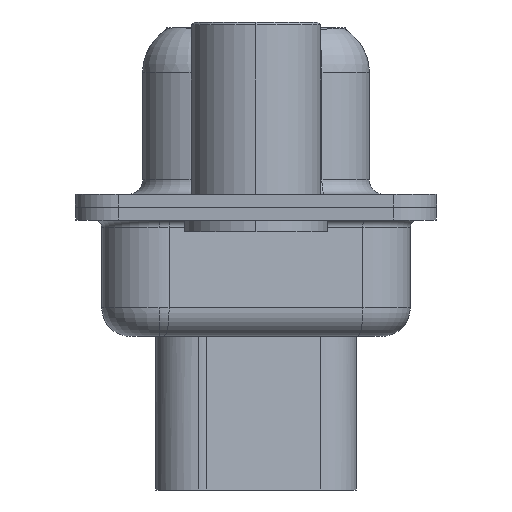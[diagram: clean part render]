
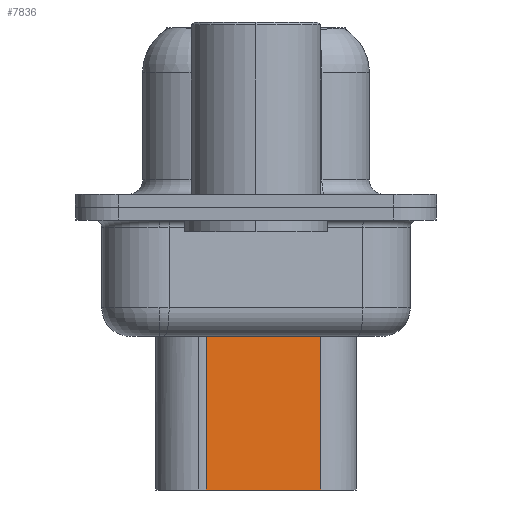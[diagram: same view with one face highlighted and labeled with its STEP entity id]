
A CAD part, left-side view. The second image highlights one B-rep face of the part: STEP entity #7836.
In plain terms, the highlighted planar face has unit normal (-0.985, -0.174, 0).
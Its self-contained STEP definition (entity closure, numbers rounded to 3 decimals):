
#334 = VECTOR ( 'NONE', #9859, 1000. ) ;
#618 = DIRECTION ( 'NONE',  ( 0.174, -0.985, 0. ) ) ;
#912 = VERTEX_POINT ( 'NONE', #12681 ) ;
#1191 = CARTESIAN_POINT ( 'NONE',  ( 5.224, -2.26, -9.85 ) ) ;
#1565 = EDGE_CURVE ( 'NONE', #13698, #3667, #4990, .T. ) ;
#1774 = LINE ( 'NONE', #20152, #334 ) ;
#2630 = ORIENTED_EDGE ( 'NONE', *, *, #1565, .F. ) ;
#2896 = EDGE_CURVE ( 'NONE', #912, #13698, #1774, .T. ) ;
#2968 = AXIS2_PLACEMENT_3D ( 'NONE', #20832, #18976, #618 ) ;
#3065 = CARTESIAN_POINT ( 'NONE',  ( 4.348, 2.709, -3.975 ) ) ;
#3270 = DIRECTION ( 'NONE',  ( -0.174, 0.985, 0. ) ) ;
#3323 = ORIENTED_EDGE ( 'NONE', *, *, #2896, .F. ) ;
#3667 = VERTEX_POINT ( 'NONE', #20899 ) ;
#4990 = LINE ( 'NONE', #23194, #18681 ) ;
#6910 = DIRECTION ( 'NONE',  ( -0.174, 0.985, 0. ) ) ;
#7495 = LINE ( 'NONE', #25951, #19107 ) ;
#7836 = ADVANCED_FACE ( 'NONE', ( #13025 ), #24889, .T. ) ;
#9026 = CARTESIAN_POINT ( 'NONE',  ( 4.519, 1.74, -3.975 ) ) ;
#9497 = EDGE_LOOP ( 'NONE', ( #3323, #19867, #20483, #2630 ) ) ;
#9859 = DIRECTION ( 'NONE',  ( 0., 0., -1. ) ) ;
#12585 = LINE ( 'NONE', #3065, #22999 ) ;
#12681 = CARTESIAN_POINT ( 'NONE',  ( 5.224, -2.26, -3.975 ) ) ;
#13025 = FACE_OUTER_BOUND ( 'NONE', #9497, .T. ) ;
#13698 = VERTEX_POINT ( 'NONE', #1191 ) ;
#16755 = EDGE_CURVE ( 'NONE', #23940, #3667, #7495, .T. ) ;
#18681 = VECTOR ( 'NONE', #3270, 1000. ) ;
#18976 = DIRECTION ( 'NONE',  ( -0.985, -0.174, 0. ) ) ;
#19107 = VECTOR ( 'NONE', #25680, 1000. ) ;
#19867 = ORIENTED_EDGE ( 'NONE', *, *, #24454, .T. ) ;
#20152 = CARTESIAN_POINT ( 'NONE',  ( 5.224, -2.26, -3.1 ) ) ;
#20483 = ORIENTED_EDGE ( 'NONE', *, *, #16755, .T. ) ;
#20832 = CARTESIAN_POINT ( 'NONE',  ( 4.519, 1.74, -3.1 ) ) ;
#20899 = CARTESIAN_POINT ( 'NONE',  ( 4.519, 1.74, -9.85 ) ) ;
#22999 = VECTOR ( 'NONE', #6910, 1000. ) ;
#23194 = CARTESIAN_POINT ( 'NONE',  ( 4.519, 1.74, -9.85 ) ) ;
#23940 = VERTEX_POINT ( 'NONE', #9026 ) ;
#24454 = EDGE_CURVE ( 'NONE', #912, #23940, #12585, .T. ) ;
#24889 = PLANE ( 'NONE',  #2968 ) ;
#25680 = DIRECTION ( 'NONE',  ( 0., 0., -1. ) ) ;
#25951 = CARTESIAN_POINT ( 'NONE',  ( 4.519, 1.74, -3.1 ) ) ;
